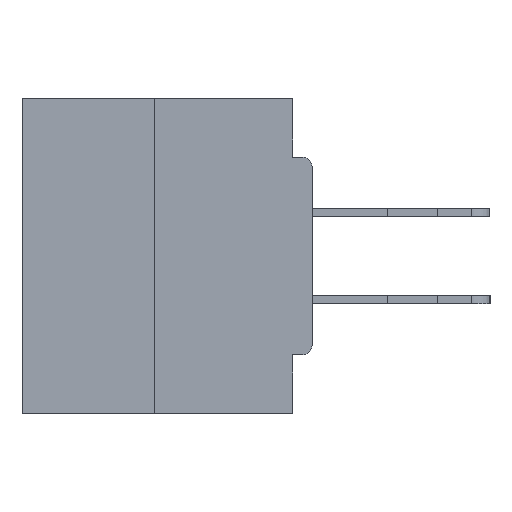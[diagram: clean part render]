
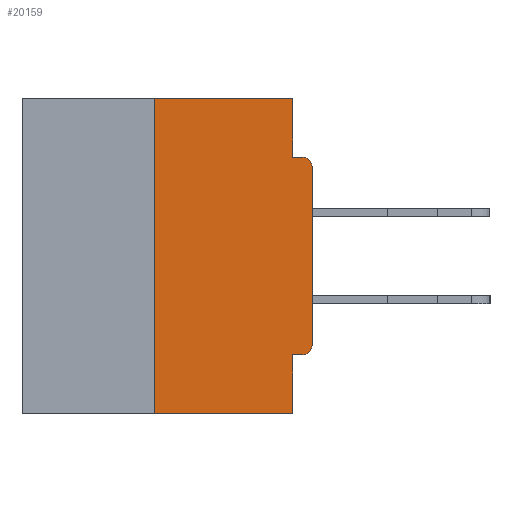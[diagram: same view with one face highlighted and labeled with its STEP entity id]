
A CAD part, left-side view. The second image highlights one B-rep face of the part: STEP entity #20159.
In plain terms, the highlighted planar face has unit normal (-1, 0, 0).
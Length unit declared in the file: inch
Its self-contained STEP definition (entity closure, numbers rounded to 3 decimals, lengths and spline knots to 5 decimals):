
#455 = CARTESIAN_POINT ( 'NONE',  ( 0., 0.25, -0.5 ) ) ;
#990 = EDGE_CURVE ( 'NONE', #29061, #34437, #13078, .T. ) ;
#1552 = AXIS2_PLACEMENT_3D ( 'NONE', #12876, #24784, #21923 ) ;
#1758 = CARTESIAN_POINT ( 'NONE',  ( 0., 0.25, 0. ) ) ;
#1974 = DIRECTION ( 'NONE',  ( 0., 1., 0. ) ) ;
#2228 = VECTOR ( 'NONE', #24778, 39.37008 ) ;
#3061 = FACE_OUTER_BOUND ( 'NONE', #26040, .T. ) ;
#3147 = CARTESIAN_POINT ( 'NONE',  ( 0., 0.46, -0.5 ) ) ;
#3188 = EDGE_CURVE ( 'NONE', #12747, #23493, #24814, .T. ) ;
#3431 = VECTOR ( 'NONE', #26942, 39.37008 ) ;
#3622 = DIRECTION ( 'NONE',  ( 0., 0., -1. ) ) ;
#3636 = AXIS2_PLACEMENT_3D ( 'NONE', #6435, #32067, #3622 ) ;
#4579 = LINE ( 'NONE', #20031, #33663 ) ;
#5997 = VERTEX_POINT ( 'NONE', #15614 ) ;
#6153 = DIRECTION ( 'NONE',  ( 0., 0., -1. ) ) ;
#6353 = CARTESIAN_POINT ( 'NONE',  ( 0., 0., -0.3915 ) ) ;
#6435 = CARTESIAN_POINT ( 'NONE',  ( 0., 0.46, 0. ) ) ;
#6782 = ORIENTED_EDGE ( 'NONE', *, *, #14800, .T. ) ;
#7126 = LINE ( 'NONE', #30514, #3431 ) ;
#7767 = ORIENTED_EDGE ( 'NONE', *, *, #28403, .F. ) ;
#7964 = CARTESIAN_POINT ( 'NONE',  ( 0., 0.031, -0.5 ) ) ;
#8742 = CIRCLE ( 'NONE', #1552, 0.015 ) ;
#9731 = CARTESIAN_POINT ( 'NONE',  ( 0., 0., 0. ) ) ;
#10111 = DIRECTION ( 'NONE',  ( 0., 0., 1. ) ) ;
#10197 = VERTEX_POINT ( 'NONE', #10501 ) ;
#10501 = CARTESIAN_POINT ( 'NONE',  ( 0., 0.015, -0.0935 ) ) ;
#11278 = CARTESIAN_POINT ( 'NONE',  ( 0., 0.25, 0. ) ) ;
#11353 = DIRECTION ( 'NONE',  ( 0., 0., -1. ) ) ;
#11383 = CARTESIAN_POINT ( 'NONE',  ( 0., 0.015, -0.1085 ) ) ;
#11927 = VERTEX_POINT ( 'NONE', #21949 ) ;
#12086 = ORIENTED_EDGE ( 'NONE', *, *, #3188, .F. ) ;
#12747 = VERTEX_POINT ( 'NONE', #34815 ) ;
#12876 = CARTESIAN_POINT ( 'NONE',  ( 0., 0.015, -0.3915 ) ) ;
#13078 = LINE ( 'NONE', #1758, #2228 ) ;
#14150 = CARTESIAN_POINT ( 'NONE',  ( 0., 0.031, -0.0935 ) ) ;
#14353 = EDGE_CURVE ( 'NONE', #34437, #5997, #7126, .T. ) ;
#14800 = EDGE_CURVE ( 'NONE', #11927, #10197, #35397, .T. ) ;
#15614 = CARTESIAN_POINT ( 'NONE',  ( 0., 0.031, 0. ) ) ;
#16139 = CARTESIAN_POINT ( 'NONE',  ( 0., 0., -0.4065 ) ) ;
#17847 = DIRECTION ( 'NONE',  ( 0., -1., 0. ) ) ;
#18066 = ORIENTED_EDGE ( 'NONE', *, *, #24251, .T. ) ;
#18187 = VERTEX_POINT ( 'NONE', #6353 ) ;
#18733 = VERTEX_POINT ( 'NONE', #7964 ) ;
#19135 = AXIS2_PLACEMENT_3D ( 'NONE', #11383, #34214, #19888 ) ;
#19888 = DIRECTION ( 'NONE',  ( 0., 0., -1. ) ) ;
#20031 = CARTESIAN_POINT ( 'NONE',  ( 0., 0.031, 0. ) ) ;
#20159 = ADVANCED_FACE ( 'NONE', ( #3061 ), #26439, .F. ) ;
#21923 = DIRECTION ( 'NONE',  ( 0., 0., -1. ) ) ;
#21949 = CARTESIAN_POINT ( 'NONE',  ( 0., 0., -0.1085 ) ) ;
#22849 = EDGE_CURVE ( 'NONE', #29061, #18733, #34837, .T. ) ;
#23424 = VECTOR ( 'NONE', #30108, 39.37008 ) ;
#23493 = VERTEX_POINT ( 'NONE', #26025 ) ;
#23677 = CARTESIAN_POINT ( 'NONE',  ( 0., 0., -0.0935 ) ) ;
#24240 = ORIENTED_EDGE ( 'NONE', *, *, #14353, .F. ) ;
#24251 = EDGE_CURVE ( 'NONE', #18187, #11927, #27270, .T. ) ;
#24778 = DIRECTION ( 'NONE',  ( 0., 0., 1. ) ) ;
#24784 = DIRECTION ( 'NONE',  ( -1., 0., 0. ) ) ;
#24814 = LINE ( 'NONE', #16139, #29605 ) ;
#24871 = EDGE_CURVE ( 'NONE', #12747, #18187, #8742, .T. ) ;
#25417 = ORIENTED_EDGE ( 'NONE', *, *, #24871, .T. ) ;
#25505 = ORIENTED_EDGE ( 'NONE', *, *, #990, .F. ) ;
#25605 = CARTESIAN_POINT ( 'NONE',  ( 0., 0.031, -0.5 ) ) ;
#25627 = VECTOR ( 'NONE', #10111, 39.37008 ) ;
#26025 = CARTESIAN_POINT ( 'NONE',  ( 0., 0.031, -0.4065 ) ) ;
#26040 = EDGE_LOOP ( 'NONE', ( #24240, #25505, #35457, #35047, #12086, #25417, #18066, #6782, #7767, #28295 ) ) ;
#26439 = PLANE ( 'NONE',  #3636 ) ;
#26942 = DIRECTION ( 'NONE',  ( 0., -1., 0. ) ) ;
#27270 = LINE ( 'NONE', #9731, #25627 ) ;
#27798 = EDGE_CURVE ( 'NONE', #5997, #35652, #4579, .T. ) ;
#28295 = ORIENTED_EDGE ( 'NONE', *, *, #27798, .F. ) ;
#28403 = EDGE_CURVE ( 'NONE', #35652, #10197, #32924, .T. ) ;
#29061 = VERTEX_POINT ( 'NONE', #455 ) ;
#29605 = VECTOR ( 'NONE', #1974, 39.37008 ) ;
#30108 = DIRECTION ( 'NONE',  ( 0., -1., 0. ) ) ;
#30415 = VECTOR ( 'NONE', #6153, 39.37008 ) ;
#30514 = CARTESIAN_POINT ( 'NONE',  ( 0., 0.46, 0. ) ) ;
#32067 = DIRECTION ( 'NONE',  ( 1., 0., 0. ) ) ;
#32797 = VECTOR ( 'NONE', #17847, 39.37008 ) ;
#32924 = LINE ( 'NONE', #23677, #23424 ) ;
#33663 = VECTOR ( 'NONE', #11353, 39.37008 ) ;
#34214 = DIRECTION ( 'NONE',  ( -1., 0., 0. ) ) ;
#34437 = VERTEX_POINT ( 'NONE', #11278 ) ;
#34457 = EDGE_CURVE ( 'NONE', #23493, #18733, #34836, .T. ) ;
#34815 = CARTESIAN_POINT ( 'NONE',  ( 0., 0.015, -0.4065 ) ) ;
#34836 = LINE ( 'NONE', #25605, #30415 ) ;
#34837 = LINE ( 'NONE', #3147, #32797 ) ;
#35047 = ORIENTED_EDGE ( 'NONE', *, *, #34457, .F. ) ;
#35397 = CIRCLE ( 'NONE', #19135, 0.015 ) ;
#35457 = ORIENTED_EDGE ( 'NONE', *, *, #22849, .T. ) ;
#35652 = VERTEX_POINT ( 'NONE', #14150 ) ;
